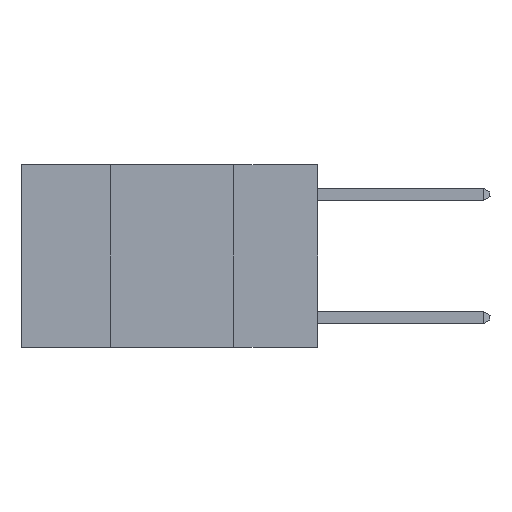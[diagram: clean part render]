
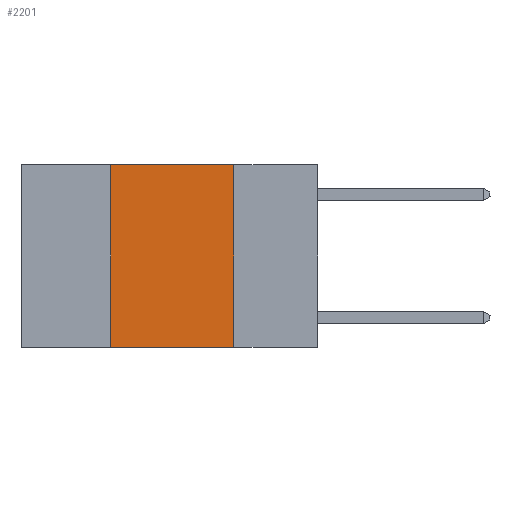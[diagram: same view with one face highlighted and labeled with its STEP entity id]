
A CAD part, left-side view. The second image highlights one B-rep face of the part: STEP entity #2201.
In plain terms, the highlighted planar face has unit normal (-1, 0, 0).
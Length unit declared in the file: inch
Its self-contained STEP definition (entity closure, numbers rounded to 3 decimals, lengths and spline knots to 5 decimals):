
#10 = EDGE_CURVE ( 'NONE', #18015, #11115, #5330, .T. ) ;
#1222 = CARTESIAN_POINT ( 'NONE',  ( 0., 0.42, 0. ) ) ;
#1406 = DIRECTION ( 'NONE',  ( 0., 0., 1. ) ) ;
#1635 = LINE ( 'NONE', #13646, #3097 ) ;
#1714 = CARTESIAN_POINT ( 'NONE',  ( 0., 0.6, 0. ) ) ;
#2201 = ADVANCED_FACE ( 'NONE', ( #3374 ), #10282, .F. ) ;
#2960 = DIRECTION ( 'NONE',  ( 0., -1., 0. ) ) ;
#3097 = VECTOR ( 'NONE', #1406, 39.37008 ) ;
#3374 = FACE_OUTER_BOUND ( 'NONE', #16325, .T. ) ;
#3757 = ORIENTED_EDGE ( 'NONE', *, *, #9808, .T. ) ;
#3913 = CARTESIAN_POINT ( 'NONE',  ( 0., 0.17, 0. ) ) ;
#3981 = VECTOR ( 'NONE', #8388, 39.37008 ) ;
#5330 = LINE ( 'NONE', #1714, #3981 ) ;
#5828 = DIRECTION ( 'NONE',  ( 0., 0., -1. ) ) ;
#7096 = DIRECTION ( 'NONE',  ( 1., 0., 0. ) ) ;
#7373 = VECTOR ( 'NONE', #12511, 39.37008 ) ;
#8388 = DIRECTION ( 'NONE',  ( 0., -1., 0. ) ) ;
#8439 = LINE ( 'NONE', #15115, #7373 ) ;
#8859 = CARTESIAN_POINT ( 'NONE',  ( 0., 0.17, -0.37 ) ) ;
#9536 = LINE ( 'NONE', #9768, #16564 ) ;
#9768 = CARTESIAN_POINT ( 'NONE',  ( 0., 0.6, -0.37 ) ) ;
#9808 = EDGE_CURVE ( 'NONE', #11996, #14252, #9536, .T. ) ;
#10282 = PLANE ( 'NONE',  #21380 ) ;
#11115 = VERTEX_POINT ( 'NONE', #3913 ) ;
#11996 = VERTEX_POINT ( 'NONE', #12455 ) ;
#12455 = CARTESIAN_POINT ( 'NONE',  ( 0., 0.42, -0.37 ) ) ;
#12511 = DIRECTION ( 'NONE',  ( 0., 0., -1. ) ) ;
#13646 = CARTESIAN_POINT ( 'NONE',  ( 0., 0.42, 0. ) ) ;
#14141 = EDGE_CURVE ( 'NONE', #11996, #18015, #1635, .T. ) ;
#14252 = VERTEX_POINT ( 'NONE', #8859 ) ;
#14781 = ORIENTED_EDGE ( 'NONE', *, *, #14141, .F. ) ;
#15115 = CARTESIAN_POINT ( 'NONE',  ( 0., 0.17, 0. ) ) ;
#15904 = CARTESIAN_POINT ( 'NONE',  ( 0., 0.6, 0. ) ) ;
#16325 = EDGE_LOOP ( 'NONE', ( #16683, #17378, #14781, #3757 ) ) ;
#16564 = VECTOR ( 'NONE', #2960, 39.37008 ) ;
#16683 = ORIENTED_EDGE ( 'NONE', *, *, #17316, .F. ) ;
#17316 = EDGE_CURVE ( 'NONE', #11115, #14252, #8439, .T. ) ;
#17378 = ORIENTED_EDGE ( 'NONE', *, *, #10, .F. ) ;
#18015 = VERTEX_POINT ( 'NONE', #1222 ) ;
#21380 = AXIS2_PLACEMENT_3D ( 'NONE', #15904, #7096, #5828 ) ;
